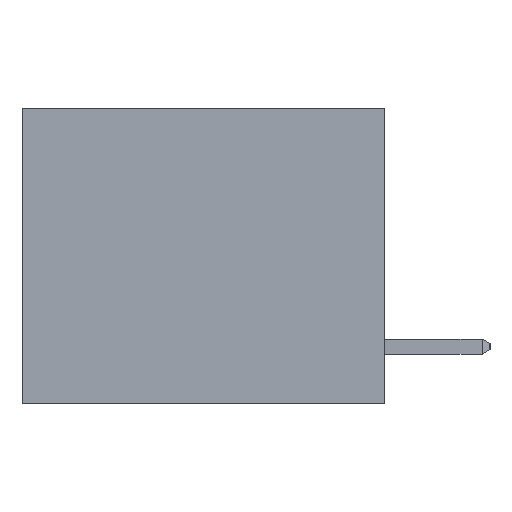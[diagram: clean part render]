
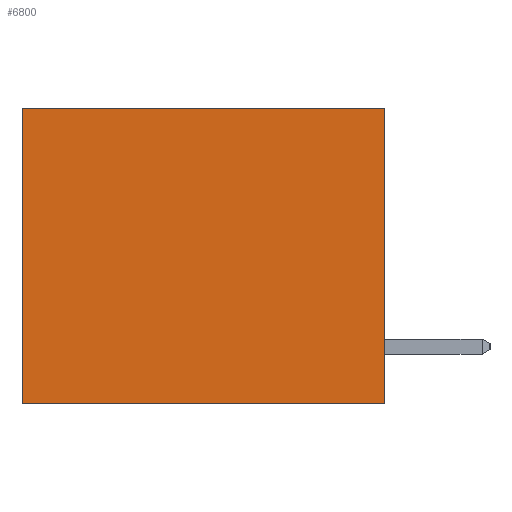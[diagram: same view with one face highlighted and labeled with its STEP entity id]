
A CAD part, left-side view. The second image highlights one B-rep face of the part: STEP entity #6800.
In plain terms, the highlighted planar face has unit normal (-1, 0, 0).
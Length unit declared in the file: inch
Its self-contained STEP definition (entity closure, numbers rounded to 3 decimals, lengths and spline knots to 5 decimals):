
#771 = EDGE_CURVE ( 'NONE', #9611, #9949, #9660, .T. ) ;
#1109 = FACE_OUTER_BOUND ( 'NONE', #10610, .T. ) ;
#1126 = ORIENTED_EDGE ( 'NONE', *, *, #8740, .F. ) ;
#1292 = VECTOR ( 'NONE', #4629, 39.37008 ) ;
#1324 = DIRECTION ( 'NONE',  ( 0., 0., -1. ) ) ;
#1726 = PLANE ( 'NONE',  #4356 ) ;
#2229 = CARTESIAN_POINT ( 'NONE',  ( 0.3165, 0., -0.49 ) ) ;
#2839 = VERTEX_POINT ( 'NONE', #10833 ) ;
#3439 = CARTESIAN_POINT ( 'NONE',  ( 0.3165, 0., 0. ) ) ;
#3462 = VECTOR ( 'NONE', #8541, 39.37008 ) ;
#3861 = CARTESIAN_POINT ( 'NONE',  ( 0.3165, 0., -0.49 ) ) ;
#4006 = ORIENTED_EDGE ( 'NONE', *, *, #7796, .T. ) ;
#4356 = AXIS2_PLACEMENT_3D ( 'NONE', #3861, #9971, #11031 ) ;
#4449 = CARTESIAN_POINT ( 'NONE',  ( 0.3165, 0., -0.49 ) ) ;
#4629 = DIRECTION ( 'NONE',  ( 0., 0., -1. ) ) ;
#5561 = VECTOR ( 'NONE', #11987, 39.37008 ) ;
#6624 = VERTEX_POINT ( 'NONE', #7756 ) ;
#6800 = ADVANCED_FACE ( 'NONE', ( #1109 ), #1726, .F. ) ;
#7460 = CARTESIAN_POINT ( 'NONE',  ( 0.3165, 0.6, -0.49 ) ) ;
#7562 = EDGE_CURVE ( 'NONE', #9611, #2839, #12271, .T. ) ;
#7756 = CARTESIAN_POINT ( 'NONE',  ( 0.3165, 0.6, -0.49 ) ) ;
#7796 = EDGE_CURVE ( 'NONE', #2839, #6624, #8831, .T. ) ;
#8541 = DIRECTION ( 'NONE',  ( 0., 1., 0. ) ) ;
#8740 = EDGE_CURVE ( 'NONE', #9949, #6624, #8975, .T. ) ;
#8759 = ORIENTED_EDGE ( 'NONE', *, *, #7562, .T. ) ;
#8831 = LINE ( 'NONE', #7460, #10440 ) ;
#8975 = LINE ( 'NONE', #4449, #3462 ) ;
#9035 = ORIENTED_EDGE ( 'NONE', *, *, #771, .F. ) ;
#9611 = VERTEX_POINT ( 'NONE', #3439 ) ;
#9660 = LINE ( 'NONE', #2229, #1292 ) ;
#9776 = CARTESIAN_POINT ( 'NONE',  ( 0.3165, 0., 0. ) ) ;
#9949 = VERTEX_POINT ( 'NONE', #13029 ) ;
#9971 = DIRECTION ( 'NONE',  ( 1., 0., 0. ) ) ;
#10440 = VECTOR ( 'NONE', #1324, 39.37008 ) ;
#10610 = EDGE_LOOP ( 'NONE', ( #4006, #1126, #9035, #8759 ) ) ;
#10833 = CARTESIAN_POINT ( 'NONE',  ( 0.3165, 0.6, 0. ) ) ;
#11031 = DIRECTION ( 'NONE',  ( 0., 0., -1. ) ) ;
#11987 = DIRECTION ( 'NONE',  ( 0., 1., 0. ) ) ;
#12271 = LINE ( 'NONE', #9776, #5561 ) ;
#13029 = CARTESIAN_POINT ( 'NONE',  ( 0.3165, 0., -0.49 ) ) ;
